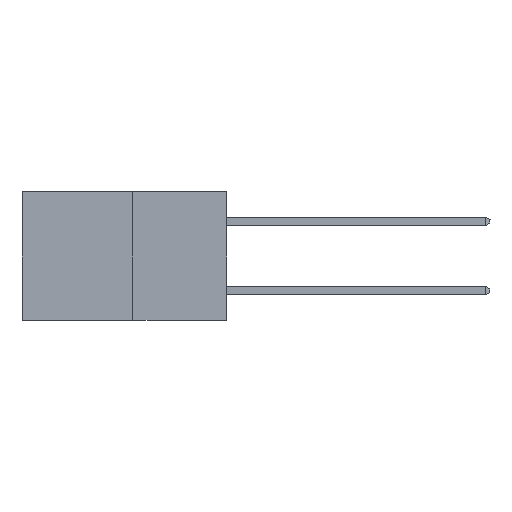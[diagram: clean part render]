
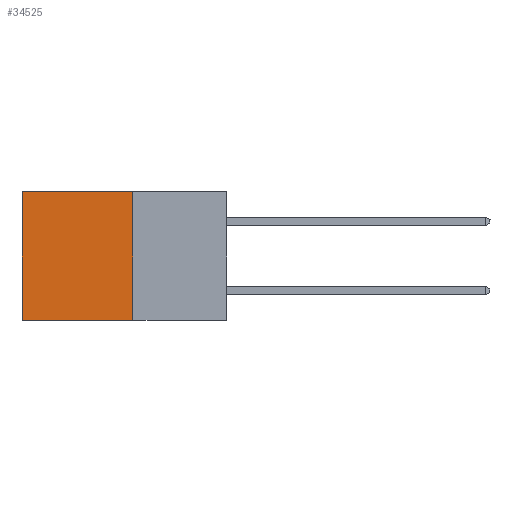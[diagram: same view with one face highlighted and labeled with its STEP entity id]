
A CAD part, left-side view. The second image highlights one B-rep face of the part: STEP entity #34525.
In plain terms, the highlighted planar face has unit normal (-1, 0, 0).
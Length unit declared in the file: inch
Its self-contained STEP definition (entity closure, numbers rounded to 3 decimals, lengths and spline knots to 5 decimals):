
#413 = CARTESIAN_POINT ( 'NONE',  ( 0.277, 0.59, -0.37 ) ) ;
#1257 = CARTESIAN_POINT ( 'NONE',  ( 0.277, 0.27, -0.37 ) ) ;
#1564 = CARTESIAN_POINT ( 'NONE',  ( 0.277, 0.59, -0.37 ) ) ;
#1958 = VERTEX_POINT ( 'NONE', #9399 ) ;
#2940 = ORIENTED_EDGE ( 'NONE', *, *, #18450, .T. ) ;
#3303 = AXIS2_PLACEMENT_3D ( 'NONE', #1257, #29014, #12393 ) ;
#5060 = LINE ( 'NONE', #27905, #26277 ) ;
#6637 = LINE ( 'NONE', #34266, #20465 ) ;
#7531 = ORIENTED_EDGE ( 'NONE', *, *, #27382, .T. ) ;
#8611 = FACE_OUTER_BOUND ( 'NONE', #23925, .T. ) ;
#9399 = CARTESIAN_POINT ( 'NONE',  ( 0.277, 0.59, 0. ) ) ;
#12086 = DIRECTION ( 'NONE',  ( 0., 0., -1. ) ) ;
#12393 = DIRECTION ( 'NONE',  ( 0., 0., -1. ) ) ;
#13754 = ORIENTED_EDGE ( 'NONE', *, *, #29094, .F. ) ;
#13795 = CARTESIAN_POINT ( 'NONE',  ( 0.277, 0.27, 0. ) ) ;
#15060 = PLANE ( 'NONE',  #3303 ) ;
#17389 = EDGE_CURVE ( 'NONE', #35572, #26270, #6637, .T. ) ;
#18169 = CARTESIAN_POINT ( 'NONE',  ( 0.277, 0.27, 0. ) ) ;
#18450 = EDGE_CURVE ( 'NONE', #1958, #22271, #29967, .T. ) ;
#20465 = VECTOR ( 'NONE', #12086, 39.37008 ) ;
#20968 = DIRECTION ( 'NONE',  ( 0., 1., 0. ) ) ;
#22271 = VERTEX_POINT ( 'NONE', #1564 ) ;
#22458 = DIRECTION ( 'NONE',  ( 0., 1., 0. ) ) ;
#22960 = LINE ( 'NONE', #18169, #29488 ) ;
#23442 = CARTESIAN_POINT ( 'NONE',  ( 0.277, 0.27, -0.37 ) ) ;
#23925 = EDGE_LOOP ( 'NONE', ( #2940, #13754, #26072, #7531 ) ) ;
#26072 = ORIENTED_EDGE ( 'NONE', *, *, #17389, .F. ) ;
#26270 = VERTEX_POINT ( 'NONE', #23442 ) ;
#26277 = VECTOR ( 'NONE', #22458, 39.37008 ) ;
#27382 = EDGE_CURVE ( 'NONE', #35572, #1958, #22960, .T. ) ;
#27905 = CARTESIAN_POINT ( 'NONE',  ( 0.277, 0.27, -0.37 ) ) ;
#29014 = DIRECTION ( 'NONE',  ( 1., 0., 0. ) ) ;
#29094 = EDGE_CURVE ( 'NONE', #26270, #22271, #5060, .T. ) ;
#29488 = VECTOR ( 'NONE', #20968, 39.37008 ) ;
#29967 = LINE ( 'NONE', #413, #35570 ) ;
#33485 = DIRECTION ( 'NONE',  ( 0., 0., -1. ) ) ;
#34266 = CARTESIAN_POINT ( 'NONE',  ( 0.277, 0.27, -0.37 ) ) ;
#34525 = ADVANCED_FACE ( 'NONE', ( #8611 ), #15060, .F. ) ;
#35570 = VECTOR ( 'NONE', #33485, 39.37008 ) ;
#35572 = VERTEX_POINT ( 'NONE', #13795 ) ;
